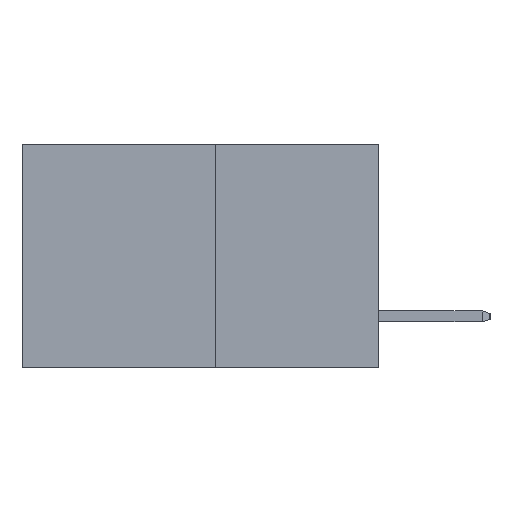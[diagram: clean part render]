
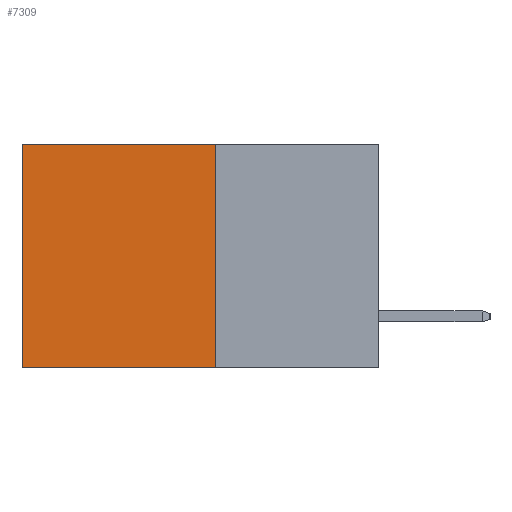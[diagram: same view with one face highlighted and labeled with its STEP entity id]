
A CAD part, left-side view. The second image highlights one B-rep face of the part: STEP entity #7309.
In plain terms, the highlighted planar face has unit normal (-1, 0, 0).
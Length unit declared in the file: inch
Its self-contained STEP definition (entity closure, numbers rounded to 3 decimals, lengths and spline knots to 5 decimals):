
#197 = EDGE_LOOP ( 'NONE', ( #7394, #2796, #1601, #3449 ) ) ;
#267 = VECTOR ( 'NONE', #9540, 39.37008 ) ;
#465 = CARTESIAN_POINT ( 'NONE',  ( 0.277, 0.59, -0.37 ) ) ;
#599 = VERTEX_POINT ( 'NONE', #3950 ) ;
#1324 = DIRECTION ( 'NONE',  ( 1., 0., 0. ) ) ;
#1601 = ORIENTED_EDGE ( 'NONE', *, *, #8651, .F. ) ;
#2038 = DIRECTION ( 'NONE',  ( 0., 0., -1. ) ) ;
#2530 = VECTOR ( 'NONE', #3106, 39.37008 ) ;
#2796 = ORIENTED_EDGE ( 'NONE', *, *, #6091, .F. ) ;
#2837 = VERTEX_POINT ( 'NONE', #5230 ) ;
#3106 = DIRECTION ( 'NONE',  ( 0., 1., 0. ) ) ;
#3449 = ORIENTED_EDGE ( 'NONE', *, *, #9421, .T. ) ;
#3653 = VECTOR ( 'NONE', #2038, 39.37008 ) ;
#3813 = CARTESIAN_POINT ( 'NONE',  ( 0.277, 0.27, -0.37 ) ) ;
#3950 = CARTESIAN_POINT ( 'NONE',  ( 0.277, 0.59, 0. ) ) ;
#3994 = CARTESIAN_POINT ( 'NONE',  ( 0.277, 0.27, -0.37 ) ) ;
#4021 = AXIS2_PLACEMENT_3D ( 'NONE', #3813, #1324, #5482 ) ;
#4503 = CARTESIAN_POINT ( 'NONE',  ( 0.277, 0.27, -0.37 ) ) ;
#4654 = PLANE ( 'NONE',  #4021 ) ;
#4804 = CARTESIAN_POINT ( 'NONE',  ( 0.277, 0.27, 0. ) ) ;
#5230 = CARTESIAN_POINT ( 'NONE',  ( 0.277, 0.27, 0. ) ) ;
#5482 = DIRECTION ( 'NONE',  ( 0., 0., -1. ) ) ;
#5897 = LINE ( 'NONE', #4503, #3653 ) ;
#6091 = EDGE_CURVE ( 'NONE', #8799, #6882, #7185, .T. ) ;
#6882 = VERTEX_POINT ( 'NONE', #8916 ) ;
#7086 = DIRECTION ( 'NONE',  ( 0., 0., -1. ) ) ;
#7185 = LINE ( 'NONE', #10237, #2530 ) ;
#7279 = LINE ( 'NONE', #465, #8838 ) ;
#7309 = ADVANCED_FACE ( 'NONE', ( #8491 ), #4654, .F. ) ;
#7394 = ORIENTED_EDGE ( 'NONE', *, *, #7884, .T. ) ;
#7884 = EDGE_CURVE ( 'NONE', #599, #6882, #7279, .T. ) ;
#8491 = FACE_OUTER_BOUND ( 'NONE', #197, .T. ) ;
#8651 = EDGE_CURVE ( 'NONE', #2837, #8799, #5897, .T. ) ;
#8799 = VERTEX_POINT ( 'NONE', #3994 ) ;
#8838 = VECTOR ( 'NONE', #7086, 39.37008 ) ;
#8916 = CARTESIAN_POINT ( 'NONE',  ( 0.277, 0.59, -0.37 ) ) ;
#8930 = LINE ( 'NONE', #4804, #267 ) ;
#9421 = EDGE_CURVE ( 'NONE', #2837, #599, #8930, .T. ) ;
#9540 = DIRECTION ( 'NONE',  ( 0., 1., 0. ) ) ;
#10237 = CARTESIAN_POINT ( 'NONE',  ( 0.277, 0.27, -0.37 ) ) ;
